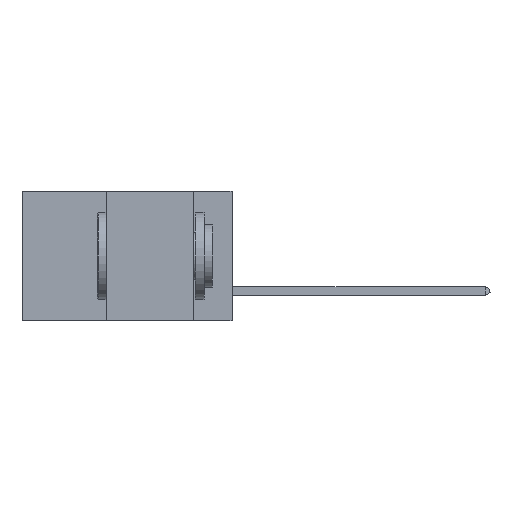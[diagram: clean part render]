
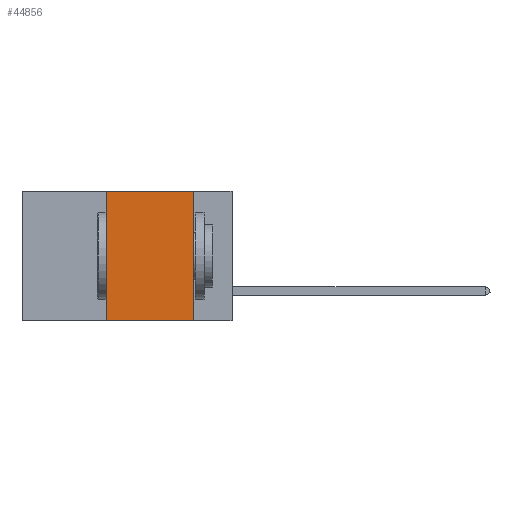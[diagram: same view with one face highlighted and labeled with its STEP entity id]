
A CAD part, left-side view. The second image highlights one B-rep face of the part: STEP entity #44856.
In plain terms, the highlighted planar face has unit normal (-1, 0, 0).
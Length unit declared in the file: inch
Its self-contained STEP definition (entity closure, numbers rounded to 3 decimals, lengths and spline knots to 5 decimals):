
#389 = LINE ( 'NONE', #29562, #9654 ) ;
#476 = AXIS2_PLACEMENT_3D ( 'NONE', #24524, #9444, #44249 ) ;
#2388 = EDGE_CURVE ( 'NONE', #36390, #23904, #17659, .T. ) ;
#4595 = CARTESIAN_POINT ( 'NONE',  ( 0., 0.6, 0. ) ) ;
#5395 = CARTESIAN_POINT ( 'NONE',  ( 0., 0.36, 0. ) ) ;
#9444 = DIRECTION ( 'NONE',  ( 1., 0., 0. ) ) ;
#9640 = EDGE_CURVE ( 'NONE', #36390, #44243, #389, .T. ) ;
#9654 = VECTOR ( 'NONE', #32608, 39.37008 ) ;
#10366 = VECTOR ( 'NONE', #24074, 39.37008 ) ;
#12865 = CARTESIAN_POINT ( 'NONE',  ( 0., 0.11, -0.37 ) ) ;
#17164 = ORIENTED_EDGE ( 'NONE', *, *, #2388, .F. ) ;
#17655 = ORIENTED_EDGE ( 'NONE', *, *, #19142, .F. ) ;
#17659 = LINE ( 'NONE', #41991, #36866 ) ;
#18940 = LINE ( 'NONE', #4595, #44653 ) ;
#19142 = EDGE_CURVE ( 'NONE', #23904, #41263, #18940, .T. ) ;
#20306 = CARTESIAN_POINT ( 'NONE',  ( 0., 0.11, 0. ) ) ;
#20522 = ORIENTED_EDGE ( 'NONE', *, *, #24422, .F. ) ;
#21027 = PLANE ( 'NONE',  #476 ) ;
#21721 = CARTESIAN_POINT ( 'NONE',  ( 0., 0.11, 0. ) ) ;
#21815 = LINE ( 'NONE', #21721, #10366 ) ;
#22470 = FACE_OUTER_BOUND ( 'NONE', #28104, .T. ) ;
#23904 = VERTEX_POINT ( 'NONE', #5395 ) ;
#24074 = DIRECTION ( 'NONE',  ( 0., 0., -1. ) ) ;
#24422 = EDGE_CURVE ( 'NONE', #41263, #44243, #21815, .T. ) ;
#24524 = CARTESIAN_POINT ( 'NONE',  ( 0., 0.6, 0. ) ) ;
#28052 = ORIENTED_EDGE ( 'NONE', *, *, #9640, .T. ) ;
#28104 = EDGE_LOOP ( 'NONE', ( #20522, #17655, #17164, #28052 ) ) ;
#29562 = CARTESIAN_POINT ( 'NONE',  ( 0., 0.6, -0.37 ) ) ;
#32608 = DIRECTION ( 'NONE',  ( 0., -1., 0. ) ) ;
#32610 = DIRECTION ( 'NONE',  ( 0., -1., 0. ) ) ;
#36390 = VERTEX_POINT ( 'NONE', #41713 ) ;
#36866 = VECTOR ( 'NONE', #38765, 39.37008 ) ;
#38765 = DIRECTION ( 'NONE',  ( 0., 0., 1. ) ) ;
#41263 = VERTEX_POINT ( 'NONE', #20306 ) ;
#41713 = CARTESIAN_POINT ( 'NONE',  ( 0., 0.36, -0.37 ) ) ;
#41991 = CARTESIAN_POINT ( 'NONE',  ( 0., 0.36, 0. ) ) ;
#44243 = VERTEX_POINT ( 'NONE', #12865 ) ;
#44249 = DIRECTION ( 'NONE',  ( 0., 0., -1. ) ) ;
#44653 = VECTOR ( 'NONE', #32610, 39.37008 ) ;
#44856 = ADVANCED_FACE ( 'NONE', ( #22470 ), #21027, .F. ) ;
